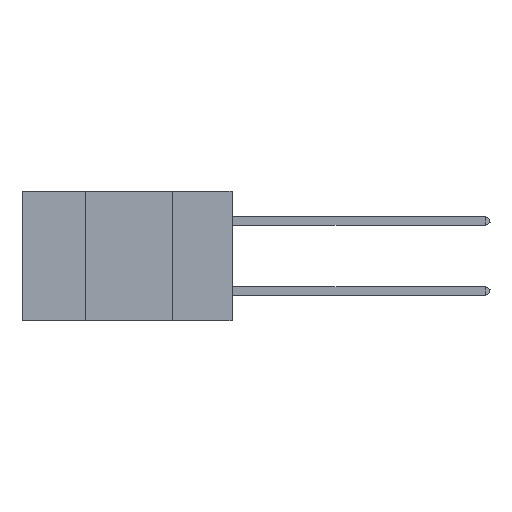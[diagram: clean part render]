
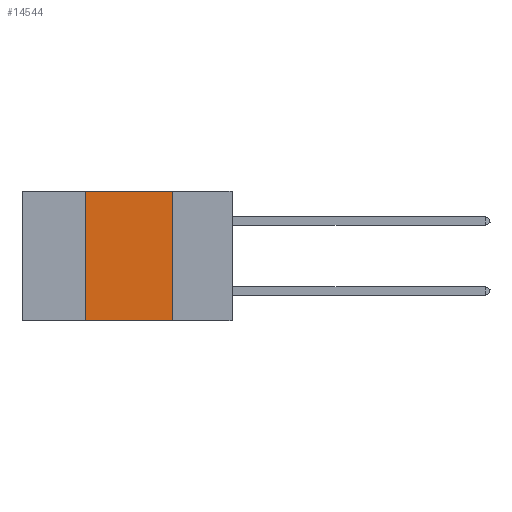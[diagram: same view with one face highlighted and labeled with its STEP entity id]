
A CAD part, left-side view. The second image highlights one B-rep face of the part: STEP entity #14544.
In plain terms, the highlighted planar face has unit normal (-1, 0, 0).
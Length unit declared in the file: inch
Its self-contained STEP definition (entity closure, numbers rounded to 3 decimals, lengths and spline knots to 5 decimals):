
#74 = FACE_OUTER_BOUND ( 'NONE', #4158, .T. ) ;
#626 = CARTESIAN_POINT ( 'NONE',  ( 0., 0.17, 0. ) ) ;
#640 = EDGE_CURVE ( 'NONE', #16321, #3096, #18252, .T. ) ;
#2616 = ORIENTED_EDGE ( 'NONE', *, *, #20620, .F. ) ;
#3096 = VERTEX_POINT ( 'NONE', #10948 ) ;
#3277 = ORIENTED_EDGE ( 'NONE', *, *, #16702, .F. ) ;
#4158 = EDGE_LOOP ( 'NONE', ( #18713, #2616, #3277, #14540 ) ) ;
#4684 = DIRECTION ( 'NONE',  ( 0., 0., 1. ) ) ;
#5475 = DIRECTION ( 'NONE',  ( 0., -1., 0. ) ) ;
#6862 = LINE ( 'NONE', #17292, #24101 ) ;
#8470 = CARTESIAN_POINT ( 'NONE',  ( 0., 0.17, 0. ) ) ;
#8560 = AXIS2_PLACEMENT_3D ( 'NONE', #24372, #12017, #26424 ) ;
#10482 = CARTESIAN_POINT ( 'NONE',  ( 0., 0.6, 0. ) ) ;
#10948 = CARTESIAN_POINT ( 'NONE',  ( 0., 0.17, -0.37 ) ) ;
#11808 = CARTESIAN_POINT ( 'NONE',  ( 0., 0.42, -0.37 ) ) ;
#12017 = DIRECTION ( 'NONE',  ( 1., 0., 0. ) ) ;
#14540 = ORIENTED_EDGE ( 'NONE', *, *, #640, .T. ) ;
#14544 = ADVANCED_FACE ( 'NONE', ( #74 ), #16144, .F. ) ;
#14807 = CARTESIAN_POINT ( 'NONE',  ( 0., 0.42, 0. ) ) ;
#15209 = LINE ( 'NONE', #10482, #26082 ) ;
#15412 = DIRECTION ( 'NONE',  ( 0., 0., -1. ) ) ;
#16144 = PLANE ( 'NONE',  #8560 ) ;
#16155 = VECTOR ( 'NONE', #15412, 39.37008 ) ;
#16321 = VERTEX_POINT ( 'NONE', #11808 ) ;
#16605 = VERTEX_POINT ( 'NONE', #8470 ) ;
#16702 = EDGE_CURVE ( 'NONE', #16321, #20022, #6862, .T. ) ;
#17292 = CARTESIAN_POINT ( 'NONE',  ( 0., 0.42, 0. ) ) ;
#18057 = CARTESIAN_POINT ( 'NONE',  ( 0., 0.6, -0.37 ) ) ;
#18252 = LINE ( 'NONE', #18057, #23056 ) ;
#18713 = ORIENTED_EDGE ( 'NONE', *, *, #20821, .F. ) ;
#20022 = VERTEX_POINT ( 'NONE', #14807 ) ;
#20620 = EDGE_CURVE ( 'NONE', #20022, #16605, #15209, .T. ) ;
#20821 = EDGE_CURVE ( 'NONE', #16605, #3096, #20966, .T. ) ;
#20966 = LINE ( 'NONE', #626, #16155 ) ;
#23056 = VECTOR ( 'NONE', #5475, 39.37008 ) ;
#24101 = VECTOR ( 'NONE', #4684, 39.37008 ) ;
#24372 = CARTESIAN_POINT ( 'NONE',  ( 0., 0.6, 0. ) ) ;
#24991 = DIRECTION ( 'NONE',  ( 0., -1., 0. ) ) ;
#26082 = VECTOR ( 'NONE', #24991, 39.37008 ) ;
#26424 = DIRECTION ( 'NONE',  ( 0., 0., -1. ) ) ;
